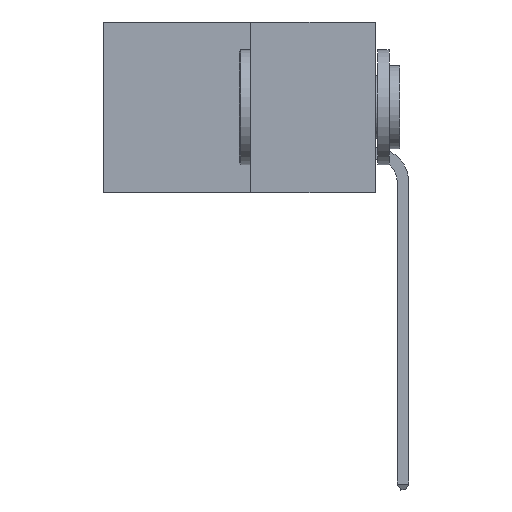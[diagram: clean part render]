
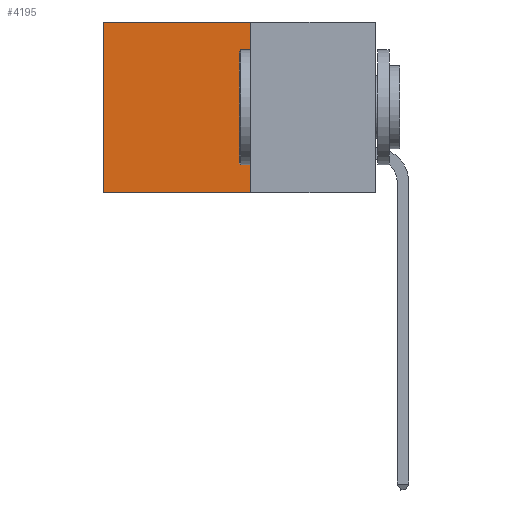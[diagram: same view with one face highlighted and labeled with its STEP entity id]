
A CAD part, left-side view. The second image highlights one B-rep face of the part: STEP entity #4195.
In plain terms, the highlighted planar face has unit normal (-1, 0, 0).
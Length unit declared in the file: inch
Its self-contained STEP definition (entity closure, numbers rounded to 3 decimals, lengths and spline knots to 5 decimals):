
#681 = VECTOR ( 'NONE', #1425, 39.37008 ) ;
#756 = DIRECTION ( 'NONE',  ( 0., 0., -1. ) ) ;
#923 = CARTESIAN_POINT ( 'NONE',  ( 0.277, 0.59, -0.37 ) ) ;
#1096 = VECTOR ( 'NONE', #5085, 39.37008 ) ;
#1425 = DIRECTION ( 'NONE',  ( 0., 0., -1. ) ) ;
#1469 = EDGE_CURVE ( 'NONE', #9964, #9710, #5735, .T. ) ;
#1580 = CARTESIAN_POINT ( 'NONE',  ( 0.277, 0.27, -0.37 ) ) ;
#1762 = FACE_OUTER_BOUND ( 'NONE', #4693, .T. ) ;
#2234 = CARTESIAN_POINT ( 'NONE',  ( 0.277, 0.27, -0.37 ) ) ;
#2423 = CARTESIAN_POINT ( 'NONE',  ( 0.277, 0.27, -0.37 ) ) ;
#3001 = DIRECTION ( 'NONE',  ( 0., 1., 0. ) ) ;
#3323 = VECTOR ( 'NONE', #3001, 39.37008 ) ;
#3868 = ORIENTED_EDGE ( 'NONE', *, *, #10354, .F. ) ;
#4195 = ADVANCED_FACE ( 'NONE', ( #1762 ), #5337, .F. ) ;
#4241 = ORIENTED_EDGE ( 'NONE', *, *, #1469, .F. ) ;
#4414 = EDGE_CURVE ( 'NONE', #8222, #9710, #6027, .T. ) ;
#4693 = EDGE_LOOP ( 'NONE', ( #8883, #4241, #3868, #9281 ) ) ;
#4717 = AXIS2_PLACEMENT_3D ( 'NONE', #5505, #5051, #4974 ) ;
#4974 = DIRECTION ( 'NONE',  ( 0., 0., -1. ) ) ;
#5051 = DIRECTION ( 'NONE',  ( 1., 0., 0. ) ) ;
#5085 = DIRECTION ( 'NONE',  ( 0., 1., 0. ) ) ;
#5128 = CARTESIAN_POINT ( 'NONE',  ( 0.277, 0.27, 0. ) ) ;
#5252 = EDGE_CURVE ( 'NONE', #7835, #8222, #7779, .T. ) ;
#5337 = PLANE ( 'NONE',  #4717 ) ;
#5505 = CARTESIAN_POINT ( 'NONE',  ( 0.277, 0.27, -0.37 ) ) ;
#5735 = LINE ( 'NONE', #2423, #3323 ) ;
#6027 = LINE ( 'NONE', #923, #8019 ) ;
#6818 = CARTESIAN_POINT ( 'NONE',  ( 0.277, 0.59, 0. ) ) ;
#7779 = LINE ( 'NONE', #5128, #1096 ) ;
#7835 = VERTEX_POINT ( 'NONE', #9555 ) ;
#7906 = LINE ( 'NONE', #2234, #681 ) ;
#8019 = VECTOR ( 'NONE', #756, 39.37008 ) ;
#8222 = VERTEX_POINT ( 'NONE', #6818 ) ;
#8883 = ORIENTED_EDGE ( 'NONE', *, *, #4414, .T. ) ;
#9281 = ORIENTED_EDGE ( 'NONE', *, *, #5252, .T. ) ;
#9529 = CARTESIAN_POINT ( 'NONE',  ( 0.277, 0.59, -0.37 ) ) ;
#9555 = CARTESIAN_POINT ( 'NONE',  ( 0.277, 0.27, 0. ) ) ;
#9710 = VERTEX_POINT ( 'NONE', #9529 ) ;
#9964 = VERTEX_POINT ( 'NONE', #1580 ) ;
#10354 = EDGE_CURVE ( 'NONE', #7835, #9964, #7906, .T. ) ;
